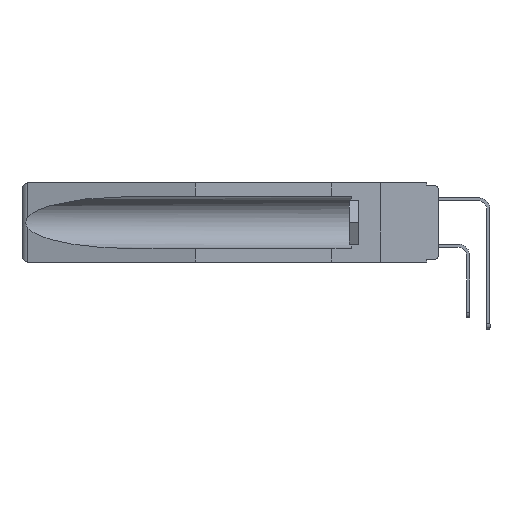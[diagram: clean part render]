
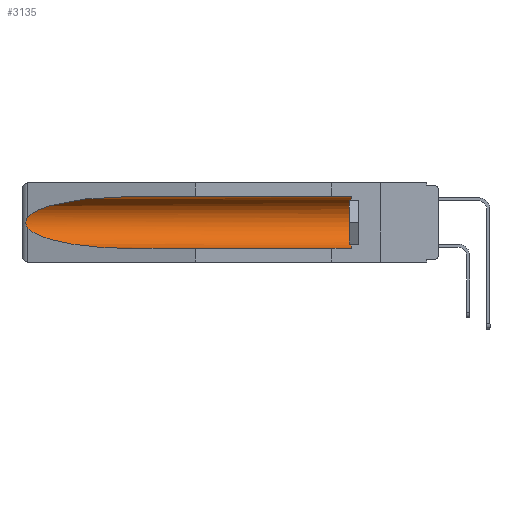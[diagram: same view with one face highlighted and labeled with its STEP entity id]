
A CAD part, left-side view. The second image highlights one B-rep face of the part: STEP entity #3135.
In plain terms, the highlighted cylindrical face has radius 2.857 mm (diameter 5.715 mm), a partial arc.
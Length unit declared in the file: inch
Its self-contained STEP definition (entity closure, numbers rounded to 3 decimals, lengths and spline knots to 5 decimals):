
#383 = CARTESIAN_POINT ( 'NONE',  ( 0.26597, 1.52961, -0.15275 ) ) ;
#677 = DIRECTION ( 'NONE',  ( 0., 1., 0. ) ) ;
#1494 = DIRECTION ( 'NONE',  ( 0., -1., 0. ) ) ;
#1583 = ORIENTED_EDGE ( 'NONE', *, *, #19749, .T. ) ;
#1889 = AXIS2_PLACEMENT_3D ( 'NONE', #11295, #1494, #11548 ) ;
#2298 = CARTESIAN_POINT ( 'NONE',  ( 0.2673, 1.53269, -0.17917 ) ) ;
#2369 = LINE ( 'NONE', #8244, #8843 ) ;
#2521 = CARTESIAN_POINT ( 'NONE',  ( 0.155, 0.126, -0.284 ) ) ;
#2602 = CARTESIAN_POINT ( 'NONE',  ( 0.21114, 1.30732, -0.059 ) ) ;
#3135 = ADVANCED_FACE ( 'NONE', ( #16335 ), #18361, .F. ) ;
#3387 = EDGE_CURVE ( 'NONE', #14860, #7671, #7286, .T. ) ;
#4035 = VERTEX_POINT ( 'NONE', #2521 ) ;
#4639 = CARTESIAN_POINT ( 'NONE',  ( 0.155, 1.07973, -0.059 ) ) ;
#4762 = CARTESIAN_POINT ( 'NONE',  ( 0.25451, 1.48313, -0.09465 ) ) ;
#4839 = EDGE_CURVE ( 'NONE', #4035, #23619, #22616, .T. ) ;
#5456 = EDGE_LOOP ( 'NONE', ( #10567, #8071, #1583, #15139, #17936, #7569 ) ) ;
#5882 = CARTESIAN_POINT ( 'NONE',  ( 0.26654, 1.53092, -0.15636 ) ) ;
#6142 = CARTESIAN_POINT ( 'NONE',  ( 0.155, 1.07973, -0.284 ) ) ;
#6359 = EDGE_CURVE ( 'NONE', #23619, #22697, #2369, .T. ) ;
#6991 = VECTOR ( 'NONE', #12478, 39.37008 ) ;
#7286 = B_SPLINE_CURVE_WITH_KNOTS ( 'NONE', 3,
 ( #23197, #383, #5882, #17456, #23458, #17717, #2298, #9825, #9692, #8158 ),
 .UNSPECIFIED., .F., .F.,
 ( 4, 2, 2, 2, 4 ),
 ( 0., 0.00029, 0.00058, 0.00087, 0.00117 ),
 .UNSPECIFIED. ) ;
#7569 = ORIENTED_EDGE ( 'NONE', *, *, #6359, .T. ) ;
#7671 = VERTEX_POINT ( 'NONE', #10400 ) ;
#8071 = ORIENTED_EDGE ( 'NONE', *, *, #3387, .T. ) ;
#8158 = CARTESIAN_POINT ( 'NONE',  ( 0.26537, 1.52718, -0.19328 ) ) ;
#8244 = CARTESIAN_POINT ( 'NONE',  ( 0.155, -0.30754, -0.059 ) ) ;
#8843 = VECTOR ( 'NONE', #15874, 39.37008 ) ;
#9692 = CARTESIAN_POINT ( 'NONE',  ( 0.26597, 1.5296, -0.19026 ) ) ;
#9825 = CARTESIAN_POINT ( 'NONE',  ( 0.26655, 1.53094, -0.18657 ) ) ;
#10400 = CARTESIAN_POINT ( 'NONE',  ( 0.26537, 1.52718, -0.19328 ) ) ;
#10567 = ORIENTED_EDGE ( 'NONE', *, *, #13513, .T. ) ;
#11295 = CARTESIAN_POINT ( 'NONE',  ( 0.155, 0.126, -0.1715 ) ) ;
#11548 = DIRECTION ( 'NONE',  ( 0., 0., 1. ) ) ;
#11650 = CARTESIAN_POINT ( 'NONE',  ( 0.26537, 1.52718, -0.14972 ) ) ;
#12243 = CARTESIAN_POINT ( 'NONE',  ( 0.155, 0.126, -0.059 ) ) ;
#12478 = DIRECTION ( 'NONE',  ( 0., 1., 0. ) ) ;
#12996 = VERTEX_POINT ( 'NONE', #6142 ) ;
#13018 = EDGE_CURVE ( 'NONE', #4035, #12996, #24099, .T. ) ;
#13513 = EDGE_CURVE ( 'NONE', #22697, #14860, #24970, .T. ) ;
#13628 = CARTESIAN_POINT ( 'NONE',  ( 0.155, 1.07973, -0.059 ) ) ;
#14860 = VERTEX_POINT ( 'NONE', #11650 ) ;
#15139 = ORIENTED_EDGE ( 'NONE', *, *, #13018, .F. ) ;
#15874 = DIRECTION ( 'NONE',  ( 0., 1., 0. ) ) ;
#16335 = FACE_OUTER_BOUND ( 'NONE', #5456, .T. ) ;
#16478 = CARTESIAN_POINT ( 'NONE',  ( 0.26537, 1.52718, -0.14972 ) ) ;
#17456 = CARTESIAN_POINT ( 'NONE',  ( 0.2673, 1.5327, -0.16383 ) ) ;
#17717 = CARTESIAN_POINT ( 'NONE',  ( 0.2675, 1.53308, -0.17534 ) ) ;
#17849 = CARTESIAN_POINT ( 'NONE',  ( 0.155, -0.30754, -0.284 ) ) ;
#17921 = CARTESIAN_POINT ( 'NONE',  ( 0.25451, 1.48313, -0.24835 ) ) ;
#17936 = ORIENTED_EDGE ( 'NONE', *, *, #4839, .T. ) ;
#18238 = CARTESIAN_POINT ( 'NONE',  ( 0.155, -0.30754, -0.1715 ) ) ;
#18361 = CYLINDRICAL_SURFACE ( 'NONE', #18421, 0.1125 ) ;
#18417 = CARTESIAN_POINT ( 'NONE',  ( 0.155, 1.07973, -0.284 ) ) ;
#18421 = AXIS2_PLACEMENT_3D ( 'NONE', #18238, #677, #24115 ) ;
#19749 = EDGE_CURVE ( 'NONE', #7671, #12996, #24149, .T. ) ;
#22116 = CARTESIAN_POINT ( 'NONE',  ( 0.21114, 1.30732, -0.284 ) ) ;
#22616 = CIRCLE ( 'NONE', #1889, 0.1125 ) ;
#22697 = VERTEX_POINT ( 'NONE', #13628 ) ;
#23197 = CARTESIAN_POINT ( 'NONE',  ( 0.26537, 1.52718, -0.14972 ) ) ;
#23458 = CARTESIAN_POINT ( 'NONE',  ( 0.2675, 1.53308, -0.16763 ) ) ;
#23619 = VERTEX_POINT ( 'NONE', #12243 ) ;
#24042 = CARTESIAN_POINT ( 'NONE',  ( 0.26537, 1.52718, -0.19328 ) ) ;
#24099 = LINE ( 'NONE', #17849, #6991 ) ;
#24115 = DIRECTION ( 'NONE',  ( 0., 0., 1. ) ) ;
#24149 =( BOUNDED_CURVE ( )  B_SPLINE_CURVE ( 3, ( #24042, #17921, #22116, #18417 ),
 .UNSPECIFIED., .F., .F. ) 
 B_SPLINE_CURVE_WITH_KNOTS ( ( 4, 4 ),
 ( 0.1948, 1.5708 ),
 .UNSPECIFIED. ) 
 CURVE ( )  GEOMETRIC_REPRESENTATION_ITEM ( )  RATIONAL_B_SPLINE_CURVE ( ( 1., 0.848, 0.848, 1. ) ) 
 REPRESENTATION_ITEM ( '' )  );
#24970 =( BOUNDED_CURVE ( )  B_SPLINE_CURVE ( 3, ( #4639, #2602, #4762, #16478 ),
 .UNSPECIFIED., .F., .F. ) 
 B_SPLINE_CURVE_WITH_KNOTS ( ( 4, 4 ),
 ( 4.71239, 6.08839 ),
 .UNSPECIFIED. ) 
 CURVE ( )  GEOMETRIC_REPRESENTATION_ITEM ( )  RATIONAL_B_SPLINE_CURVE ( ( 1., 0.848, 0.848, 1. ) ) 
 REPRESENTATION_ITEM ( '' )  );
